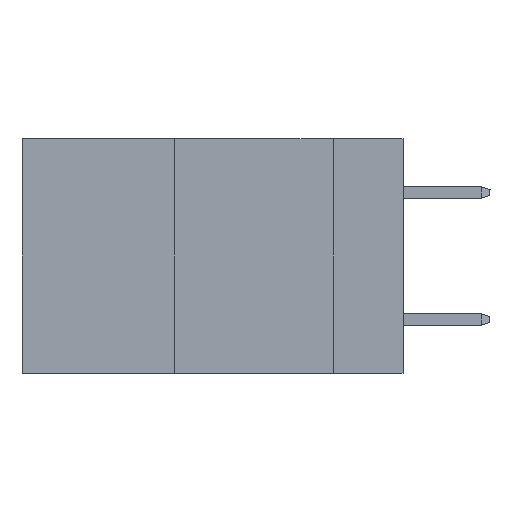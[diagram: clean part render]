
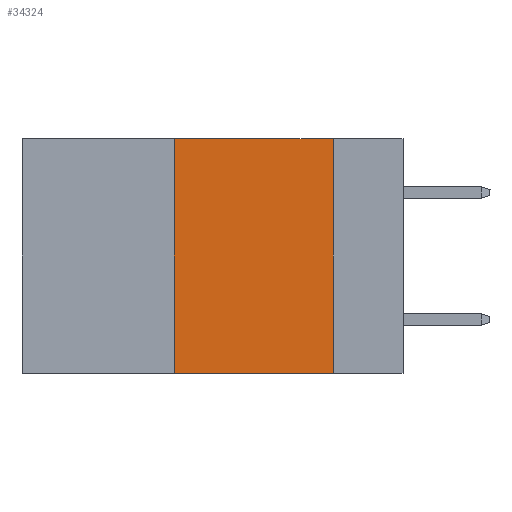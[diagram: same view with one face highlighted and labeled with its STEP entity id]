
A CAD part, left-side view. The second image highlights one B-rep face of the part: STEP entity #34324.
In plain terms, the highlighted planar face has unit normal (-1, 0, 0).
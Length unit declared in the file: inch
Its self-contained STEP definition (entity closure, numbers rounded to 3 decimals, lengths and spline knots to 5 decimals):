
#262 = CARTESIAN_POINT ( 'NONE',  ( 0., 0.6, 0. ) ) ;
#460 = CARTESIAN_POINT ( 'NONE',  ( 0., 0.36, 0. ) ) ;
#2012 = EDGE_LOOP ( 'NONE', ( #13577, #21654, #4404, #16099 ) ) ;
#2985 = PLANE ( 'NONE',  #25917 ) ;
#3985 = EDGE_CURVE ( 'NONE', #12485, #11975, #37255, .T. ) ;
#4404 = ORIENTED_EDGE ( 'NONE', *, *, #27146, .F. ) ;
#4433 = CARTESIAN_POINT ( 'NONE',  ( 0., 0.11, 0. ) ) ;
#4563 = CARTESIAN_POINT ( 'NONE',  ( 0., 0.36, 0. ) ) ;
#5138 = EDGE_CURVE ( 'NONE', #16053, #37088, #27694, .T. ) ;
#5384 = CARTESIAN_POINT ( 'NONE',  ( 0., 0.6, -0.37 ) ) ;
#7394 = DIRECTION ( 'NONE',  ( 0., 0., 1. ) ) ;
#7546 = CARTESIAN_POINT ( 'NONE',  ( 0., 0.36, -0.37 ) ) ;
#7891 = CARTESIAN_POINT ( 'NONE',  ( 0., 0.11, 0. ) ) ;
#9287 = DIRECTION ( 'NONE',  ( 0., -1., 0. ) ) ;
#9351 = DIRECTION ( 'NONE',  ( 0., 0., -1. ) ) ;
#10720 = VECTOR ( 'NONE', #7394, 39.37008 ) ;
#11384 = VECTOR ( 'NONE', #38332, 39.37008 ) ;
#11975 = VERTEX_POINT ( 'NONE', #7891 ) ;
#12485 = VERTEX_POINT ( 'NONE', #4563 ) ;
#12600 = FACE_OUTER_BOUND ( 'NONE', #2012, .T. ) ;
#13577 = ORIENTED_EDGE ( 'NONE', *, *, #26232, .F. ) ;
#16053 = VERTEX_POINT ( 'NONE', #7546 ) ;
#16099 = ORIENTED_EDGE ( 'NONE', *, *, #5138, .T. ) ;
#16896 = LINE ( 'NONE', #4433, #11384 ) ;
#21654 = ORIENTED_EDGE ( 'NONE', *, *, #3985, .F. ) ;
#25303 = CARTESIAN_POINT ( 'NONE',  ( 0., 0.6, 0. ) ) ;
#25917 = AXIS2_PLACEMENT_3D ( 'NONE', #25303, #34671, #9351 ) ;
#26232 = EDGE_CURVE ( 'NONE', #11975, #37088, #16896, .T. ) ;
#27146 = EDGE_CURVE ( 'NONE', #16053, #12485, #37853, .T. ) ;
#27489 = VECTOR ( 'NONE', #9287, 39.37008 ) ;
#27568 = VECTOR ( 'NONE', #30148, 39.37008 ) ;
#27694 = LINE ( 'NONE', #5384, #27568 ) ;
#30148 = DIRECTION ( 'NONE',  ( 0., -1., 0. ) ) ;
#31270 = CARTESIAN_POINT ( 'NONE',  ( 0., 0.11, -0.37 ) ) ;
#34324 = ADVANCED_FACE ( 'NONE', ( #12600 ), #2985, .F. ) ;
#34671 = DIRECTION ( 'NONE',  ( 1., 0., 0. ) ) ;
#37088 = VERTEX_POINT ( 'NONE', #31270 ) ;
#37255 = LINE ( 'NONE', #262, #27489 ) ;
#37853 = LINE ( 'NONE', #460, #10720 ) ;
#38332 = DIRECTION ( 'NONE',  ( 0., 0., -1. ) ) ;
